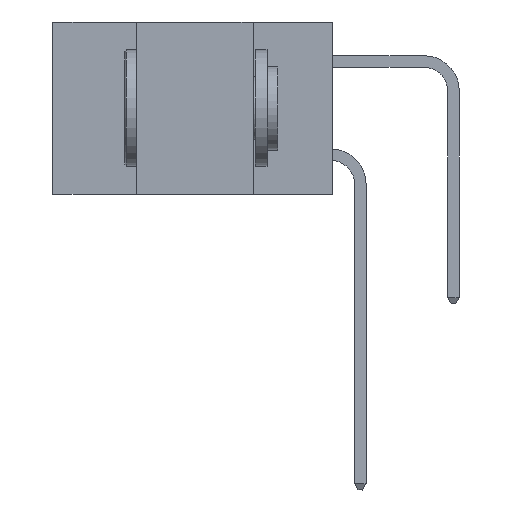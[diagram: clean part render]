
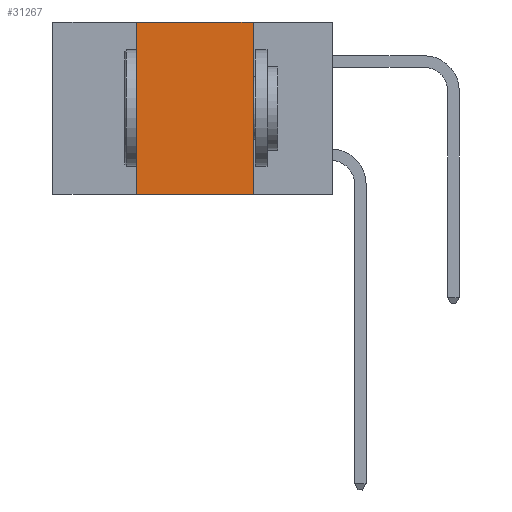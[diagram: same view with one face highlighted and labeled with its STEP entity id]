
A CAD part, left-side view. The second image highlights one B-rep face of the part: STEP entity #31267.
In plain terms, the highlighted planar face has unit normal (-1, 0, 0).
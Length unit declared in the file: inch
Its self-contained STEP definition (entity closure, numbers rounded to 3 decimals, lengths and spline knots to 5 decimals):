
#682 = CARTESIAN_POINT ( 'NONE',  ( 0., 0.6, -0.37 ) ) ;
#2828 = VECTOR ( 'NONE', #19738, 39.37008 ) ;
#2861 = ORIENTED_EDGE ( 'NONE', *, *, #5974, .F. ) ;
#4394 = ORIENTED_EDGE ( 'NONE', *, *, #4740, .T. ) ;
#4453 = VERTEX_POINT ( 'NONE', #18861 ) ;
#4584 = PLANE ( 'NONE',  #25369 ) ;
#4740 = EDGE_CURVE ( 'NONE', #4453, #13459, #11123, .T. ) ;
#5372 = EDGE_CURVE ( 'NONE', #15483, #13459, #23961, .T. ) ;
#5974 = EDGE_CURVE ( 'NONE', #4453, #21254, #19207, .T. ) ;
#6052 = CARTESIAN_POINT ( 'NONE',  ( 0., 0.17, 0. ) ) ;
#7272 = CARTESIAN_POINT ( 'NONE',  ( 0., 0.6, 0. ) ) ;
#9521 = CARTESIAN_POINT ( 'NONE',  ( 0., 0.6, 0. ) ) ;
#11123 = LINE ( 'NONE', #682, #16985 ) ;
#11556 = ORIENTED_EDGE ( 'NONE', *, *, #12389, .F. ) ;
#11917 = LINE ( 'NONE', #7272, #2828 ) ;
#12389 = EDGE_CURVE ( 'NONE', #21254, #15483, #11917, .T. ) ;
#13459 = VERTEX_POINT ( 'NONE', #30207 ) ;
#14283 = DIRECTION ( 'NONE',  ( 0., 0., -1. ) ) ;
#15483 = VERTEX_POINT ( 'NONE', #6052 ) ;
#15859 = EDGE_LOOP ( 'NONE', ( #18583, #11556, #2861, #4394 ) ) ;
#16784 = DIRECTION ( 'NONE',  ( 0., 0., 1. ) ) ;
#16985 = VECTOR ( 'NONE', #18616, 39.37008 ) ;
#17269 = CARTESIAN_POINT ( 'NONE',  ( 0., 0.42, 0. ) ) ;
#18583 = ORIENTED_EDGE ( 'NONE', *, *, #5372, .F. ) ;
#18616 = DIRECTION ( 'NONE',  ( 0., -1., 0. ) ) ;
#18861 = CARTESIAN_POINT ( 'NONE',  ( 0., 0.42, -0.37 ) ) ;
#19207 = LINE ( 'NONE', #24327, #31060 ) ;
#19738 = DIRECTION ( 'NONE',  ( 0., -1., 0. ) ) ;
#20039 = VECTOR ( 'NONE', #25167, 39.37008 ) ;
#21254 = VERTEX_POINT ( 'NONE', #17269 ) ;
#22128 = DIRECTION ( 'NONE',  ( 1., 0., 0. ) ) ;
#22516 = CARTESIAN_POINT ( 'NONE',  ( 0., 0.17, 0. ) ) ;
#23961 = LINE ( 'NONE', #22516, #20039 ) ;
#24327 = CARTESIAN_POINT ( 'NONE',  ( 0., 0.42, 0. ) ) ;
#25167 = DIRECTION ( 'NONE',  ( 0., 0., -1. ) ) ;
#25369 = AXIS2_PLACEMENT_3D ( 'NONE', #9521, #22128, #14283 ) ;
#27079 = FACE_OUTER_BOUND ( 'NONE', #15859, .T. ) ;
#30207 = CARTESIAN_POINT ( 'NONE',  ( 0., 0.17, -0.37 ) ) ;
#31060 = VECTOR ( 'NONE', #16784, 39.37008 ) ;
#31267 = ADVANCED_FACE ( 'NONE', ( #27079 ), #4584, .F. ) ;
